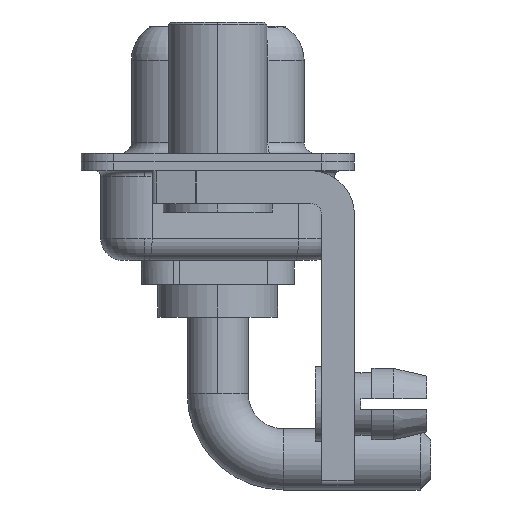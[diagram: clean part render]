
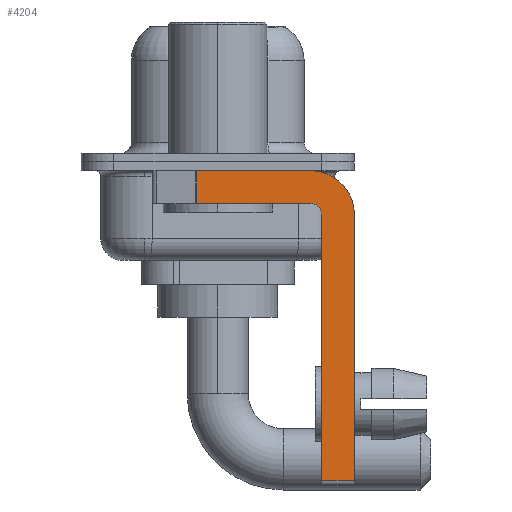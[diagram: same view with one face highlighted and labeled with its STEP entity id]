
A CAD part, left-side view. The second image highlights one B-rep face of the part: STEP entity #4204.
In plain terms, the highlighted planar face has unit normal (-1, 0, 0).
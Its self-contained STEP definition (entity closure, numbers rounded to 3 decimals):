
#206 = LINE ( 'NONE', #8321, #3396 ) ;
#345 = LINE ( 'NONE', #1708, #1783 ) ;
#472 = EDGE_CURVE ( 'NONE', #15051, #7253, #5890, .T. ) ;
#776 = EDGE_LOOP ( 'NONE', ( #7015, #6285, #5917, #9755, #6263, #10558, #4154, #1073 ) ) ;
#1073 = ORIENTED_EDGE ( 'NONE', *, *, #472, .F. ) ;
#1506 = CARTESIAN_POINT ( 'NONE',  ( -2.9, -4.75, -14.55 ) ) ;
#1708 = CARTESIAN_POINT ( 'NONE',  ( -2.9, -6.25, -2.4 ) ) ;
#1783 = VECTOR ( 'NONE', #9410, 1000. ) ;
#2593 = CARTESIAN_POINT ( 'NONE',  ( -2.9, -4.75, -2.4 ) ) ;
#2882 = AXIS2_PLACEMENT_3D ( 'NONE', #9898, #3315, #12447 ) ;
#3315 = DIRECTION ( 'NONE',  ( 1., 0., 0. ) ) ;
#3396 = VECTOR ( 'NONE', #5589, 1000. ) ;
#3417 = AXIS2_PLACEMENT_3D ( 'NONE', #15062, #16195, #7055 ) ;
#3619 = EDGE_CURVE ( 'NONE', #4991, #10556, #5990, .T. ) ;
#3654 = CARTESIAN_POINT ( 'NONE',  ( -2.9, -6.25, -14.55 ) ) ;
#3664 = AXIS2_PLACEMENT_3D ( 'NONE', #4169, #14604, #13308 ) ;
#3996 = CARTESIAN_POINT ( 'NONE',  ( -2.9, -4.25, -1.9 ) ) ;
#4154 = ORIENTED_EDGE ( 'NONE', *, *, #4178, .F. ) ;
#4169 = CARTESIAN_POINT ( 'NONE',  ( -2.9, -4.25, -2.4 ) ) ;
#4178 = EDGE_CURVE ( 'NONE', #7253, #15448, #345, .T. ) ;
#4204 = ADVANCED_FACE ( 'NONE', ( #10657 ), #8112, .F. ) ;
#4244 = EDGE_CURVE ( 'NONE', #7060, #10556, #206, .T. ) ;
#4991 = VERTEX_POINT ( 'NONE', #16733 ) ;
#5002 = CARTESIAN_POINT ( 'NONE',  ( -2.9, 0.978, -1.9 ) ) ;
#5157 = EDGE_CURVE ( 'NONE', #4991, #15051, #9594, .T. ) ;
#5589 = DIRECTION ( 'NONE',  ( 0., 1., 0. ) ) ;
#5766 = CARTESIAN_POINT ( 'NONE',  ( -2.9, -4.25, -0.4 ) ) ;
#5890 = CIRCLE ( 'NONE', #2882, 2. ) ;
#5917 = ORIENTED_EDGE ( 'NONE', *, *, #4244, .F. ) ;
#5990 = LINE ( 'NONE', #9838, #11661 ) ;
#6263 = ORIENTED_EDGE ( 'NONE', *, *, #12606, .F. ) ;
#6285 = ORIENTED_EDGE ( 'NONE', *, *, #3619, .T. ) ;
#6496 = LINE ( 'NONE', #12209, #10366 ) ;
#6664 = VECTOR ( 'NONE', #15284, 1000. ) ;
#6915 = DIRECTION ( 'NONE',  ( 0., -1., 0. ) ) ;
#7015 = ORIENTED_EDGE ( 'NONE', *, *, #5157, .F. ) ;
#7055 = DIRECTION ( 'NONE',  ( 0., 0., 1. ) ) ;
#7060 = VERTEX_POINT ( 'NONE', #3996 ) ;
#7253 = VERTEX_POINT ( 'NONE', #8531 ) ;
#7437 = CARTESIAN_POINT ( 'NONE',  ( -2.9, -4.25, -14.55 ) ) ;
#8089 = EDGE_CURVE ( 'NONE', #11242, #15448, #16419, .T. ) ;
#8112 = PLANE ( 'NONE',  #3664 ) ;
#8321 = CARTESIAN_POINT ( 'NONE',  ( -2.9, -4.25, -1.9 ) ) ;
#8511 = VECTOR ( 'NONE', #6915, 1000. ) ;
#8531 = CARTESIAN_POINT ( 'NONE',  ( -2.9, -6.25, -2.4 ) ) ;
#9410 = DIRECTION ( 'NONE',  ( 0., 0., -1. ) ) ;
#9517 = CARTESIAN_POINT ( 'NONE',  ( -2.9, 3., -0.4 ) ) ;
#9594 = LINE ( 'NONE', #9517, #8511 ) ;
#9755 = ORIENTED_EDGE ( 'NONE', *, *, #11830, .F. ) ;
#9838 = CARTESIAN_POINT ( 'NONE',  ( -2.9, 0.978, -1.9 ) ) ;
#9898 = CARTESIAN_POINT ( 'NONE',  ( -2.9, -4.25, -2.4 ) ) ;
#10366 = VECTOR ( 'NONE', #16129, 1000. ) ;
#10556 = VERTEX_POINT ( 'NONE', #5002 ) ;
#10558 = ORIENTED_EDGE ( 'NONE', *, *, #8089, .T. ) ;
#10657 = FACE_OUTER_BOUND ( 'NONE', #776, .T. ) ;
#11054 = CIRCLE ( 'NONE', #3417, 0.5 ) ;
#11242 = VERTEX_POINT ( 'NONE', #1506 ) ;
#11661 = VECTOR ( 'NONE', #15023, 1000. ) ;
#11830 = EDGE_CURVE ( 'NONE', #14814, #7060, #11054, .T. ) ;
#12209 = CARTESIAN_POINT ( 'NONE',  ( -2.9, -4.75, -14.8 ) ) ;
#12447 = DIRECTION ( 'NONE',  ( 0., 0., -1. ) ) ;
#12606 = EDGE_CURVE ( 'NONE', #11242, #14814, #6496, .T. ) ;
#13308 = DIRECTION ( 'NONE',  ( 0., 0., -1. ) ) ;
#14604 = DIRECTION ( 'NONE',  ( 1., 0., 0. ) ) ;
#14814 = VERTEX_POINT ( 'NONE', #2593 ) ;
#15023 = DIRECTION ( 'NONE',  ( 0., 0., -1. ) ) ;
#15051 = VERTEX_POINT ( 'NONE', #5766 ) ;
#15062 = CARTESIAN_POINT ( 'NONE',  ( -2.9, -4.25, -2.4 ) ) ;
#15284 = DIRECTION ( 'NONE',  ( 0., -1., 0. ) ) ;
#15448 = VERTEX_POINT ( 'NONE', #3654 ) ;
#16129 = DIRECTION ( 'NONE',  ( 0., 0., 1. ) ) ;
#16195 = DIRECTION ( 'NONE',  ( -1., 0., 0. ) ) ;
#16419 = LINE ( 'NONE', #7437, #6664 ) ;
#16733 = CARTESIAN_POINT ( 'NONE',  ( -2.9, 0.978, -0.4 ) ) ;
